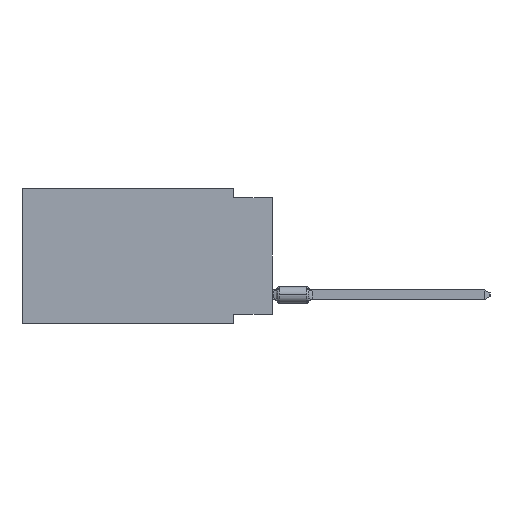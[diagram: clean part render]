
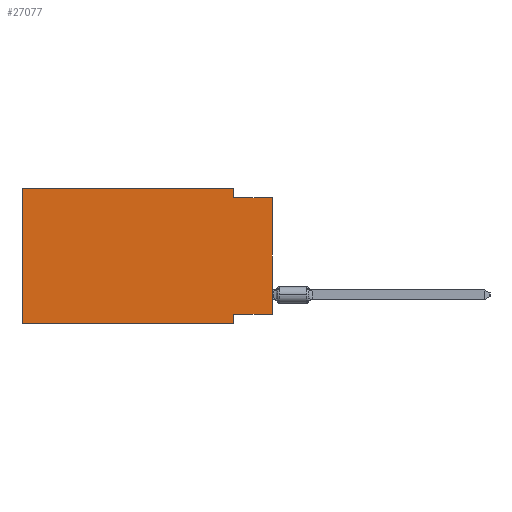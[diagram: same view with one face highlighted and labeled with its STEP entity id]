
A CAD part, left-side view. The second image highlights one B-rep face of the part: STEP entity #27077.
In plain terms, the highlighted planar face has unit normal (-1, 0, 0).
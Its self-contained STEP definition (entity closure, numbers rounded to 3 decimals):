
#542 = PLANE ( 'NONE',  #48843 ) ;
#832 = LINE ( 'NONE', #4312, #47874 ) ;
#1813 = LINE ( 'NONE', #36282, #9965 ) ;
#2256 = EDGE_CURVE ( 'NONE', #13015, #4405, #12636, .T. ) ;
#3712 = CARTESIAN_POINT ( 'NONE',  ( 0., 0., -0.635 ) ) ;
#4312 = CARTESIAN_POINT ( 'NONE',  ( 0., 16.383, 0. ) ) ;
#4405 = VERTEX_POINT ( 'NONE', #50223 ) ;
#5767 = VERTEX_POINT ( 'NONE', #21514 ) ;
#5928 = EDGE_CURVE ( 'NONE', #48303, #55134, #14572, .T. ) ;
#6377 = CARTESIAN_POINT ( 'NONE',  ( 0., 2.54, -8.255 ) ) ;
#8088 = CARTESIAN_POINT ( 'NONE',  ( 0., 2.54, -0.635 ) ) ;
#8369 = CARTESIAN_POINT ( 'NONE',  ( 0., 2.54, -8.89 ) ) ;
#8612 = VECTOR ( 'NONE', #45277, 1000. ) ;
#8816 = VERTEX_POINT ( 'NONE', #33919 ) ;
#9032 = DIRECTION ( 'NONE',  ( 0., 0., 1. ) ) ;
#9965 = VECTOR ( 'NONE', #40597, 1000. ) ;
#10099 = EDGE_CURVE ( 'NONE', #43708, #48303, #1813, .T. ) ;
#12636 = LINE ( 'NONE', #3712, #24879 ) ;
#13015 = VERTEX_POINT ( 'NONE', #8088 ) ;
#13229 = DIRECTION ( 'NONE',  ( 0., 0., 1. ) ) ;
#14057 = DIRECTION ( 'NONE',  ( 0., 0., -1. ) ) ;
#14337 = CARTESIAN_POINT ( 'NONE',  ( 0., 16.383, 0. ) ) ;
#14572 = LINE ( 'NONE', #24035, #8612 ) ;
#17074 = VECTOR ( 'NONE', #9032, 1000. ) ;
#18327 = LINE ( 'NONE', #31501, #50594 ) ;
#19032 = CARTESIAN_POINT ( 'NONE',  ( 0., 16.383, 0. ) ) ;
#19320 = DIRECTION ( 'NONE',  ( 0., -1., 0. ) ) ;
#19835 = ORIENTED_EDGE ( 'NONE', *, *, #2256, .F. ) ;
#19867 = EDGE_CURVE ( 'NONE', #8816, #13015, #24307, .T. ) ;
#19892 = LINE ( 'NONE', #19032, #38302 ) ;
#21514 = CARTESIAN_POINT ( 'NONE',  ( 0., 16.383, -8.89 ) ) ;
#22095 = EDGE_CURVE ( 'NONE', #43708, #4405, #30852, .T. ) ;
#23566 = EDGE_LOOP ( 'NONE', ( #25073, #19835, #46773, #39920, #36618, #56192, #46434, #26169 ) ) ;
#23726 = VERTEX_POINT ( 'NONE', #34214 ) ;
#24035 = CARTESIAN_POINT ( 'NONE',  ( 0., 2.54, -8.89 ) ) ;
#24307 = LINE ( 'NONE', #28890, #39918 ) ;
#24879 = VECTOR ( 'NONE', #39287, 1000. ) ;
#25073 = ORIENTED_EDGE ( 'NONE', *, *, #22095, .T. ) ;
#26169 = ORIENTED_EDGE ( 'NONE', *, *, #10099, .F. ) ;
#27077 = ADVANCED_FACE ( 'NONE', ( #53377 ), #542, .F. ) ;
#28890 = CARTESIAN_POINT ( 'NONE',  ( 0., 2.54, 0. ) ) ;
#30852 = LINE ( 'NONE', #52951, #17074 ) ;
#31501 = CARTESIAN_POINT ( 'NONE',  ( 0., 16.383, -8.89 ) ) ;
#32832 = CARTESIAN_POINT ( 'NONE',  ( 0., 0., -8.255 ) ) ;
#33919 = CARTESIAN_POINT ( 'NONE',  ( 0., 2.54, 0. ) ) ;
#34214 = CARTESIAN_POINT ( 'NONE',  ( 0., 16.383, 0. ) ) ;
#36282 = CARTESIAN_POINT ( 'NONE',  ( 0., 0., -8.255 ) ) ;
#36618 = ORIENTED_EDGE ( 'NONE', *, *, #56157, .F. ) ;
#38302 = VECTOR ( 'NONE', #19320, 1000. ) ;
#39287 = DIRECTION ( 'NONE',  ( 0., -1., 0. ) ) ;
#39918 = VECTOR ( 'NONE', #46405, 1000. ) ;
#39920 = ORIENTED_EDGE ( 'NONE', *, *, #48203, .F. ) ;
#40448 = DIRECTION ( 'NONE',  ( 1., 0., 0. ) ) ;
#40597 = DIRECTION ( 'NONE',  ( 0., 1., 0. ) ) ;
#43708 = VERTEX_POINT ( 'NONE', #32832 ) ;
#45277 = DIRECTION ( 'NONE',  ( 0., 0., -1. ) ) ;
#46405 = DIRECTION ( 'NONE',  ( 0., 0., -1. ) ) ;
#46434 = ORIENTED_EDGE ( 'NONE', *, *, #5928, .F. ) ;
#46773 = ORIENTED_EDGE ( 'NONE', *, *, #19867, .F. ) ;
#47450 = EDGE_CURVE ( 'NONE', #5767, #55134, #18327, .T. ) ;
#47874 = VECTOR ( 'NONE', #13229, 1000. ) ;
#48203 = EDGE_CURVE ( 'NONE', #23726, #8816, #19892, .T. ) ;
#48303 = VERTEX_POINT ( 'NONE', #6377 ) ;
#48843 = AXIS2_PLACEMENT_3D ( 'NONE', #14337, #40448, #14057 ) ;
#49014 = DIRECTION ( 'NONE',  ( 0., -1., 0. ) ) ;
#50223 = CARTESIAN_POINT ( 'NONE',  ( 0., 0., -0.635 ) ) ;
#50594 = VECTOR ( 'NONE', #49014, 1000. ) ;
#52951 = CARTESIAN_POINT ( 'NONE',  ( 0., 0., 0. ) ) ;
#53377 = FACE_OUTER_BOUND ( 'NONE', #23566, .T. ) ;
#55134 = VERTEX_POINT ( 'NONE', #8369 ) ;
#56157 = EDGE_CURVE ( 'NONE', #5767, #23726, #832, .T. ) ;
#56192 = ORIENTED_EDGE ( 'NONE', *, *, #47450, .T. ) ;
